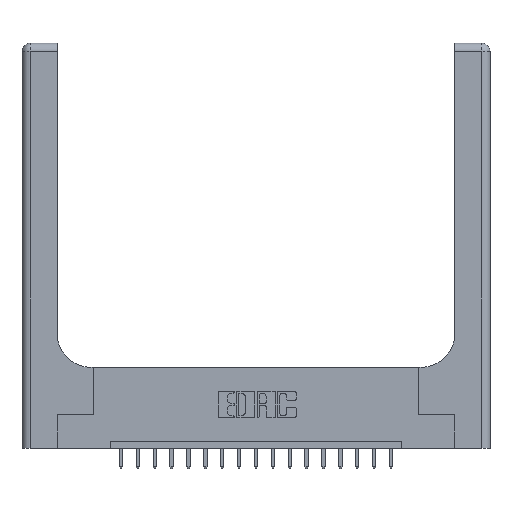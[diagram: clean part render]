
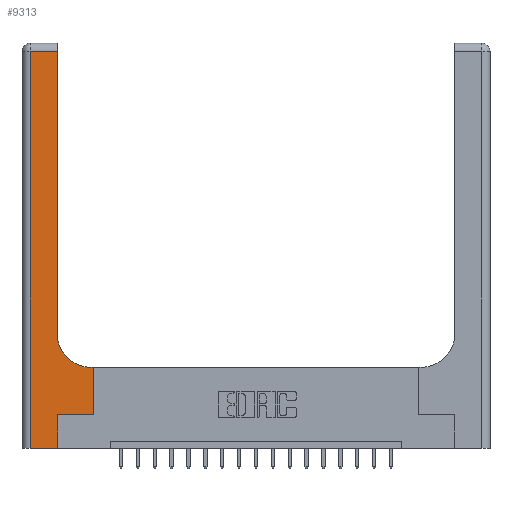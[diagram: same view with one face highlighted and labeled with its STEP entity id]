
A CAD part, top view. The second image highlights one B-rep face of the part: STEP entity #9313.
In plain terms, the highlighted planar face has unit normal (0, 0, 1).
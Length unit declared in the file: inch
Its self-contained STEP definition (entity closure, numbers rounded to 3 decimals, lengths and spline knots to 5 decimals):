
#109 = DIRECTION ( 'NONE',  ( 0., 1., 0. ) ) ;
#188 = LINE ( 'NONE', #8384, #14243 ) ;
#231 = VERTEX_POINT ( 'NONE', #7843 ) ;
#659 = VERTEX_POINT ( 'NONE', #714 ) ;
#714 = CARTESIAN_POINT ( 'NONE',  ( 0.265, 0., 0.37 ) ) ;
#848 = AXIS2_PLACEMENT_3D ( 'NONE', #7122, #17514, #1318 ) ;
#1318 = DIRECTION ( 'NONE',  ( 1., 0., 0. ) ) ;
#1495 = VERTEX_POINT ( 'NONE', #5038 ) ;
#1870 = VECTOR ( 'NONE', #13793, 39.37008 ) ;
#1941 = CARTESIAN_POINT ( 'NONE',  ( 0.06, 0., 0.37 ) ) ;
#1963 = ORIENTED_EDGE ( 'NONE', *, *, #8955, .T. ) ;
#1991 = CARTESIAN_POINT ( 'NONE',  ( 0., 0., 0.37 ) ) ;
#2022 = LINE ( 'NONE', #15711, #11733 ) ;
#2738 = CARTESIAN_POINT ( 'NONE',  ( 0.26, 3., 0.37 ) ) ;
#2828 = VERTEX_POINT ( 'NONE', #16296 ) ;
#3181 = CARTESIAN_POINT ( 'NONE',  ( 0., 2.94, 0.37 ) ) ;
#3608 = ORIENTED_EDGE ( 'NONE', *, *, #10368, .T. ) ;
#3786 = CARTESIAN_POINT ( 'NONE',  ( 0.06, 3., 0.37 ) ) ;
#4207 = ORIENTED_EDGE ( 'NONE', *, *, #14317, .T. ) ;
#4555 = AXIS2_PLACEMENT_3D ( 'NONE', #17539, #10145, #17471 ) ;
#4815 = VERTEX_POINT ( 'NONE', #16518 ) ;
#4965 = EDGE_CURVE ( 'NONE', #15727, #1495, #18419, .T. ) ;
#5038 = CARTESIAN_POINT ( 'NONE',  ( 0.528, 0.6, 0.37 ) ) ;
#5393 = ORIENTED_EDGE ( 'NONE', *, *, #7655, .T. ) ;
#6244 = DIRECTION ( 'NONE',  ( -1., 0., 0. ) ) ;
#6710 = DIRECTION ( 'NONE',  ( 0., -1., 0. ) ) ;
#6919 = CARTESIAN_POINT ( 'NONE',  ( 0.26, 0.85, 0.37 ) ) ;
#7122 = CARTESIAN_POINT ( 'NONE',  ( 0.51, 0.85, 0.37 ) ) ;
#7246 = CARTESIAN_POINT ( 'NONE',  ( 0.06, 2.94, 0.37 ) ) ;
#7655 = EDGE_CURVE ( 'NONE', #1495, #2828, #16277, .T. ) ;
#7671 = LINE ( 'NONE', #3786, #8585 ) ;
#7685 = DIRECTION ( 'NONE',  ( -1., 0., 0. ) ) ;
#7843 = CARTESIAN_POINT ( 'NONE',  ( 0.26, 2.94, 0.37 ) ) ;
#7982 = EDGE_CURVE ( 'NONE', #2828, #10411, #10703, .T. ) ;
#8243 = LINE ( 'NONE', #1991, #1870 ) ;
#8384 = CARTESIAN_POINT ( 'NONE',  ( 0.265, 0.25, 0.37 ) ) ;
#8585 = VECTOR ( 'NONE', #6710, 39.37008 ) ;
#8847 = EDGE_CURVE ( 'NONE', #4815, #15727, #188, .T. ) ;
#8955 = EDGE_CURVE ( 'NONE', #231, #11821, #9038, .T. ) ;
#9038 = LINE ( 'NONE', #3181, #13447 ) ;
#9313 = ADVANCED_FACE ( 'NONE', ( #13178 ), #11640, .F. ) ;
#9666 = ORIENTED_EDGE ( 'NONE', *, *, #4965, .T. ) ;
#9930 = CARTESIAN_POINT ( 'NONE',  ( 0.528, 0.25, 0.37 ) ) ;
#10145 = DIRECTION ( 'NONE',  ( 0., 0., -1. ) ) ;
#10368 = EDGE_CURVE ( 'NONE', #11821, #14272, #7671, .T. ) ;
#10394 = ORIENTED_EDGE ( 'NONE', *, *, #7982, .T. ) ;
#10411 = VERTEX_POINT ( 'NONE', #6919 ) ;
#10565 = CARTESIAN_POINT ( 'NONE',  ( 0.26, 0.6, 0.37 ) ) ;
#10703 = CIRCLE ( 'NONE', #848, 0.25 ) ;
#11640 = PLANE ( 'NONE',  #4555 ) ;
#11690 = DIRECTION ( 'NONE',  ( 0., 1., 0. ) ) ;
#11733 = VECTOR ( 'NONE', #109, 39.37008 ) ;
#11821 = VERTEX_POINT ( 'NONE', #7246 ) ;
#11884 = VECTOR ( 'NONE', #7685, 39.37008 ) ;
#12077 = ORIENTED_EDGE ( 'NONE', *, *, #8847, .T. ) ;
#12834 = EDGE_CURVE ( 'NONE', #14272, #659, #8243, .T. ) ;
#13178 = FACE_OUTER_BOUND ( 'NONE', #18931, .T. ) ;
#13447 = VECTOR ( 'NONE', #6244, 39.37008 ) ;
#13793 = DIRECTION ( 'NONE',  ( 1., 0., 0. ) ) ;
#14243 = VECTOR ( 'NONE', #18951, 39.37008 ) ;
#14272 = VERTEX_POINT ( 'NONE', #1941 ) ;
#14317 = EDGE_CURVE ( 'NONE', #659, #4815, #2022, .T. ) ;
#15426 = LINE ( 'NONE', #2738, #15879 ) ;
#15711 = CARTESIAN_POINT ( 'NONE',  ( 0.265, 0., 0.37 ) ) ;
#15727 = VERTEX_POINT ( 'NONE', #18590 ) ;
#15748 = ORIENTED_EDGE ( 'NONE', *, *, #18927, .T. ) ;
#15879 = VECTOR ( 'NONE', #11690, 39.37008 ) ;
#16277 = LINE ( 'NONE', #10565, #11884 ) ;
#16296 = CARTESIAN_POINT ( 'NONE',  ( 0.51, 0.6, 0.37 ) ) ;
#16518 = CARTESIAN_POINT ( 'NONE',  ( 0.265, 0.25, 0.37 ) ) ;
#16594 = VECTOR ( 'NONE', #18678, 39.37008 ) ;
#17471 = DIRECTION ( 'NONE',  ( -1., 0., 0. ) ) ;
#17514 = DIRECTION ( 'NONE',  ( 0., 0., -1. ) ) ;
#17539 = CARTESIAN_POINT ( 'NONE',  ( 0., 3., 0.37 ) ) ;
#18162 = ORIENTED_EDGE ( 'NONE', *, *, #12834, .T. ) ;
#18419 = LINE ( 'NONE', #9930, #16594 ) ;
#18590 = CARTESIAN_POINT ( 'NONE',  ( 0.528, 0.25, 0.37 ) ) ;
#18678 = DIRECTION ( 'NONE',  ( 0., 1., 0. ) ) ;
#18927 = EDGE_CURVE ( 'NONE', #10411, #231, #15426, .T. ) ;
#18931 = EDGE_LOOP ( 'NONE', ( #15748, #1963, #3608, #18162, #4207, #12077, #9666, #5393, #10394 ) ) ;
#18951 = DIRECTION ( 'NONE',  ( 1., 0., 0. ) ) ;
